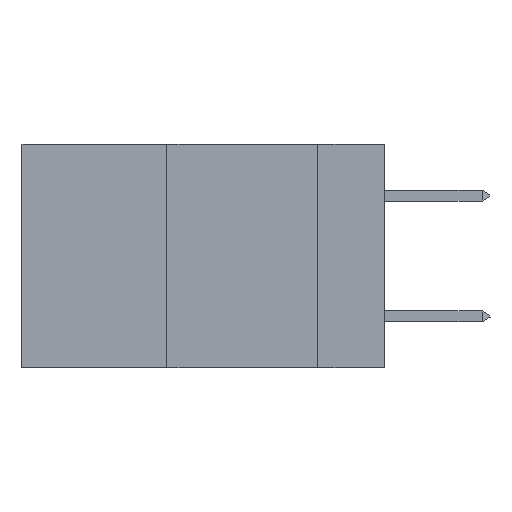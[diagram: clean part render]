
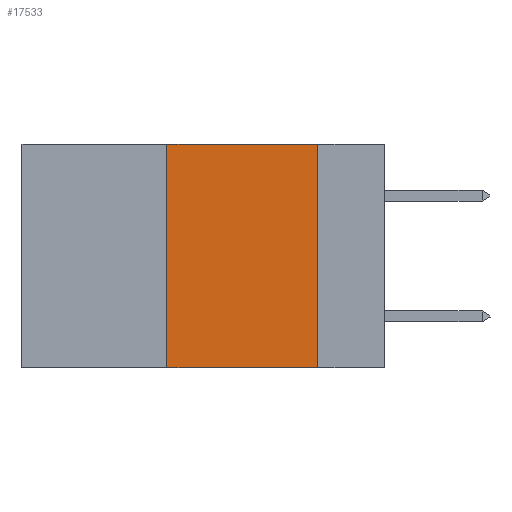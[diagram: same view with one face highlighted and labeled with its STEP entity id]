
A CAD part, left-side view. The second image highlights one B-rep face of the part: STEP entity #17533.
In plain terms, the highlighted planar face has unit normal (-1, 0, 0).
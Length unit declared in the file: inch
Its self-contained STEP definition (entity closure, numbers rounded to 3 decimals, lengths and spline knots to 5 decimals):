
#142 = VECTOR ( 'NONE', #13949, 39.37008 ) ;
#674 = FACE_OUTER_BOUND ( 'NONE', #3484, .T. ) ;
#1116 = ORIENTED_EDGE ( 'NONE', *, *, #13887, .F. ) ;
#1319 = PLANE ( 'NONE',  #4527 ) ;
#1330 = CARTESIAN_POINT ( 'NONE',  ( 0., 0.6, -0.37 ) ) ;
#1608 = CARTESIAN_POINT ( 'NONE',  ( 0., 0.36, 0. ) ) ;
#3145 = DIRECTION ( 'NONE',  ( 0., 0., -1. ) ) ;
#3354 = CARTESIAN_POINT ( 'NONE',  ( 0., 0.36, -0.37 ) ) ;
#3484 = EDGE_LOOP ( 'NONE', ( #16362, #1116, #13099, #12684 ) ) ;
#3921 = EDGE_CURVE ( 'NONE', #21831, #15286, #9595, .T. ) ;
#4527 = AXIS2_PLACEMENT_3D ( 'NONE', #11858, #13640, #3145 ) ;
#6785 = CARTESIAN_POINT ( 'NONE',  ( 0., 0.36, 0. ) ) ;
#8426 = VERTEX_POINT ( 'NONE', #22086 ) ;
#8606 = EDGE_CURVE ( 'NONE', #21831, #11622, #9813, .T. ) ;
#9595 = LINE ( 'NONE', #1330, #142 ) ;
#9752 = CARTESIAN_POINT ( 'NONE',  ( 0., 0.11, 0. ) ) ;
#9813 = LINE ( 'NONE', #1608, #17950 ) ;
#9880 = VECTOR ( 'NONE', #11462, 39.37008 ) ;
#10426 = LINE ( 'NONE', #9752, #9880 ) ;
#11462 = DIRECTION ( 'NONE',  ( 0., 0., -1. ) ) ;
#11622 = VERTEX_POINT ( 'NONE', #6785 ) ;
#11858 = CARTESIAN_POINT ( 'NONE',  ( 0., 0.6, 0. ) ) ;
#12684 = ORIENTED_EDGE ( 'NONE', *, *, #3921, .T. ) ;
#13099 = ORIENTED_EDGE ( 'NONE', *, *, #8606, .F. ) ;
#13291 = EDGE_CURVE ( 'NONE', #8426, #15286, #10426, .T. ) ;
#13640 = DIRECTION ( 'NONE',  ( 1., 0., 0. ) ) ;
#13887 = EDGE_CURVE ( 'NONE', #11622, #8426, #19890, .T. ) ;
#13949 = DIRECTION ( 'NONE',  ( 0., -1., 0. ) ) ;
#15286 = VERTEX_POINT ( 'NONE', #20231 ) ;
#16362 = ORIENTED_EDGE ( 'NONE', *, *, #13291, .F. ) ;
#16475 = CARTESIAN_POINT ( 'NONE',  ( 0., 0.6, 0. ) ) ;
#17533 = ADVANCED_FACE ( 'NONE', ( #674 ), #1319, .F. ) ;
#17950 = VECTOR ( 'NONE', #19114, 39.37008 ) ;
#18214 = DIRECTION ( 'NONE',  ( 0., -1., 0. ) ) ;
#19114 = DIRECTION ( 'NONE',  ( 0., 0., 1. ) ) ;
#19336 = VECTOR ( 'NONE', #18214, 39.37008 ) ;
#19890 = LINE ( 'NONE', #16475, #19336 ) ;
#20231 = CARTESIAN_POINT ( 'NONE',  ( 0., 0.11, -0.37 ) ) ;
#21831 = VERTEX_POINT ( 'NONE', #3354 ) ;
#22086 = CARTESIAN_POINT ( 'NONE',  ( 0., 0.11, 0. ) ) ;
